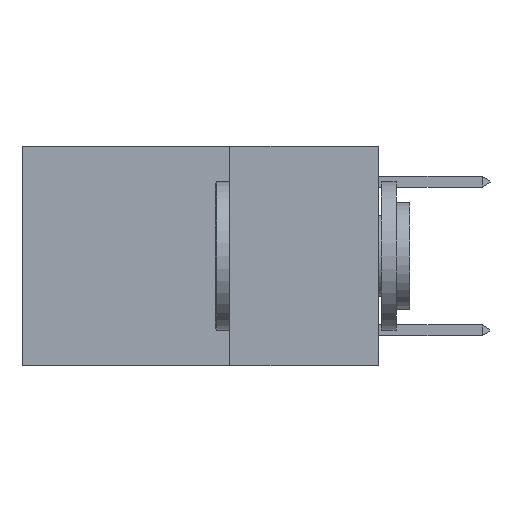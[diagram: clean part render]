
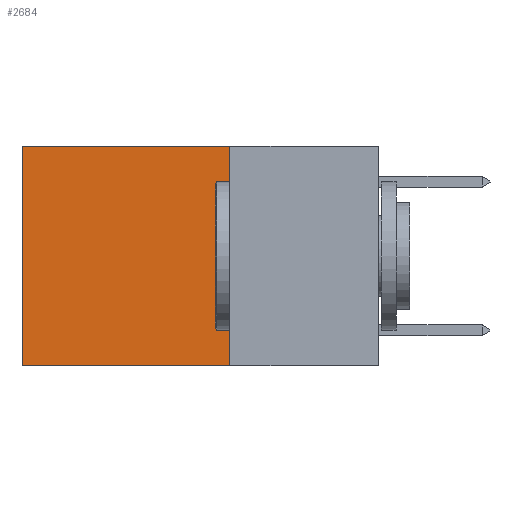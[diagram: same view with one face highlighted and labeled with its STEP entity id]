
A CAD part, left-side view. The second image highlights one B-rep face of the part: STEP entity #2684.
In plain terms, the highlighted planar face has unit normal (-1, 0, 0).
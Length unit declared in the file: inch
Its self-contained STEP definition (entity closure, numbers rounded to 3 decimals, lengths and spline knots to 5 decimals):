
#500 = PLANE ( 'NONE',  #4215 ) ;
#618 = VERTEX_POINT ( 'NONE', #20428 ) ;
#619 = DIRECTION ( 'NONE',  ( 1., 0., 0. ) ) ;
#2684 = ADVANCED_FACE ( 'NONE', ( #4893 ), #500, .F. ) ;
#3612 = EDGE_CURVE ( 'NONE', #6596, #618, #18480, .T. ) ;
#4215 = AXIS2_PLACEMENT_3D ( 'NONE', #24020, #619, #4636 ) ;
#4636 = DIRECTION ( 'NONE',  ( 0., 0., -1. ) ) ;
#4666 = DIRECTION ( 'NONE',  ( 0., 1., 0. ) ) ;
#4793 = CARTESIAN_POINT ( 'NONE',  ( 0.2625, 0.25, -0.37 ) ) ;
#4893 = FACE_OUTER_BOUND ( 'NONE', #19084, .T. ) ;
#6383 = LINE ( 'NONE', #12317, #25097 ) ;
#6596 = VERTEX_POINT ( 'NONE', #7689 ) ;
#7689 = CARTESIAN_POINT ( 'NONE',  ( 0.2625, 0.25, -0.37 ) ) ;
#8072 = CARTESIAN_POINT ( 'NONE',  ( 0.2625, 0.25, 0. ) ) ;
#11869 = CARTESIAN_POINT ( 'NONE',  ( 0.2625, 0.25, 0. ) ) ;
#12317 = CARTESIAN_POINT ( 'NONE',  ( 0.2625, 0.6, 0. ) ) ;
#14938 = VERTEX_POINT ( 'NONE', #18164 ) ;
#15786 = ORIENTED_EDGE ( 'NONE', *, *, #16726, .T. ) ;
#16063 = DIRECTION ( 'NONE',  ( 0., 0., -1. ) ) ;
#16726 = EDGE_CURVE ( 'NONE', #16975, #618, #6383, .T. ) ;
#16975 = VERTEX_POINT ( 'NONE', #21350 ) ;
#17939 = ORIENTED_EDGE ( 'NONE', *, *, #21684, .F. ) ;
#18164 = CARTESIAN_POINT ( 'NONE',  ( 0.2625, 0.25, 0. ) ) ;
#18425 = ORIENTED_EDGE ( 'NONE', *, *, #3612, .F. ) ;
#18480 = LINE ( 'NONE', #4793, #19278 ) ;
#19084 = EDGE_LOOP ( 'NONE', ( #15786, #18425, #17939, #23200 ) ) ;
#19278 = VECTOR ( 'NONE', #4666, 39.37008 ) ;
#19953 = LINE ( 'NONE', #8072, #21981 ) ;
#20080 = DIRECTION ( 'NONE',  ( 0., 1., 0. ) ) ;
#20251 = LINE ( 'NONE', #11869, #22763 ) ;
#20428 = CARTESIAN_POINT ( 'NONE',  ( 0.2625, 0.6, -0.37 ) ) ;
#21350 = CARTESIAN_POINT ( 'NONE',  ( 0.2625, 0.6, 0. ) ) ;
#21684 = EDGE_CURVE ( 'NONE', #14938, #6596, #20251, .T. ) ;
#21981 = VECTOR ( 'NONE', #20080, 39.37008 ) ;
#22763 = VECTOR ( 'NONE', #24021, 39.37008 ) ;
#23200 = ORIENTED_EDGE ( 'NONE', *, *, #23299, .T. ) ;
#23299 = EDGE_CURVE ( 'NONE', #14938, #16975, #19953, .T. ) ;
#24020 = CARTESIAN_POINT ( 'NONE',  ( 0.2625, 0.25, 0. ) ) ;
#24021 = DIRECTION ( 'NONE',  ( 0., 0., -1. ) ) ;
#25097 = VECTOR ( 'NONE', #16063, 39.37008 ) ;
